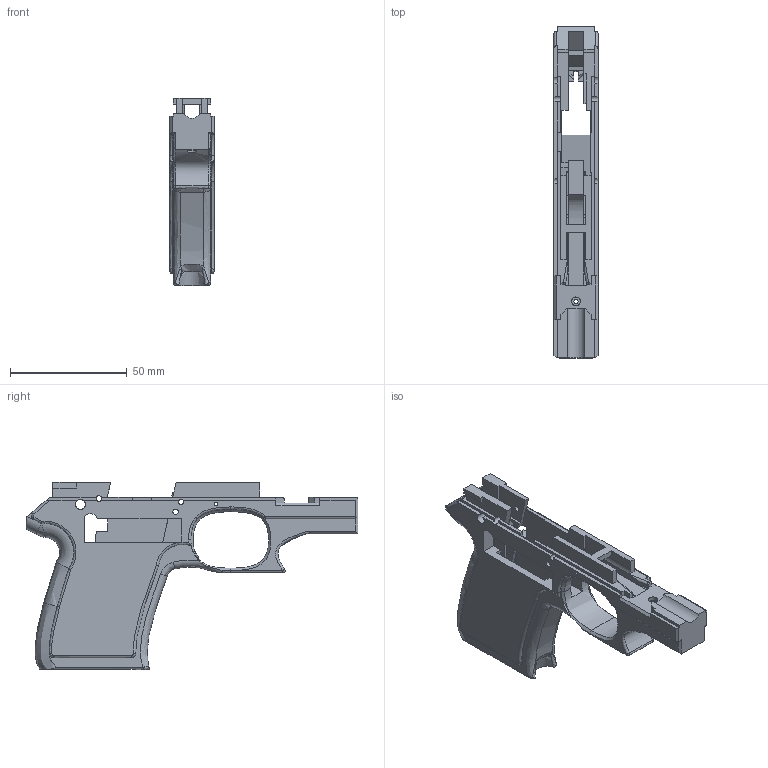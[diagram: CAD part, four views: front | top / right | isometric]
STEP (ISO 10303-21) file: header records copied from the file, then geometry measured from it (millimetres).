
FILE_DESCRIPTION(/* description */ (''),/* implementation_level */ '2;1');
FILE_NAME(/* name */ 'HP22A Type A Extractor v3.step',/* time_stamp */ '2020-02-11T23:53:23-05:00',/* author */ (''),/* organization */ (''),/* preprocessor_version */ 'ST-DEVELOPER v18',/* originating_system */ 'Autodesk Translation Framework v8.12.0.6',/* authorisation */ '');
FILE_SCHEMA (('AUTOMOTIVE_DESIGN { 1 0 10303 214 3 1 1 }'));
Length unit declared in the file: millimetre
Products named in the file (1): HP22A Type A Extractor
Bounding box: 18.9 x 142 x 80 mm (x, y, z)
Volume: 53440.7 mm3; surface area: 28046.1 mm2
Topology: 1 solids, 1 shells, 367 faces, 1035 edges, 652 vertices
Faces by surface type: plane 200, bspline 89, cylinder 60, torus 10, sphere 6, cone 2
Full cylindrical faces by diameter (mm): 1.5 x2, 1.8 x1, 2.3 x5, 2.45 x2, 3.85 x2, 4.25 x2, 5 x1, 5.7 x1, 5.75 x1
Entity records: 15282 total; most frequent: CARTESIAN_POINT 6285, ORIENTED_EDGE 2066, DIRECTION 1580, EDGE_CURVE 1033, VERTEX_POINT 652, LINE 640, VECTOR 640, AXIS2_PLACEMENT_3D 470
